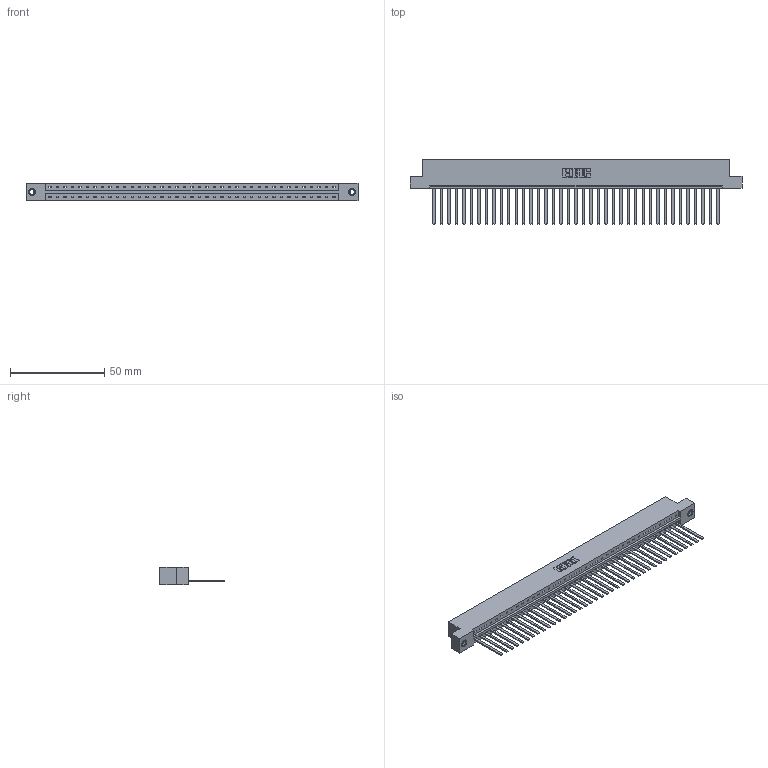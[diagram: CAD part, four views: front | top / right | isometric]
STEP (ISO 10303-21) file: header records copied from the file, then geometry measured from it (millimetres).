
FILE_DESCRIPTION (( 'STEP AP203' ), '1' );
FILE_NAME ('333-039-544-108.STEP', '2018-08-03T13:06:28', ( '' ), ( '' ), 'SwSTEP 2.0', 'SolidWorks 2016', '' );
FILE_SCHEMA (( 'CONFIG_CONTROL_DESIGN' ));
Length unit declared in the file: inch
Products named in the file (4): 333 Part_Flush - .156 Dia - TI; 345-292-001_345-293-144; 345-250-001_345-250-003-102; 333-039-544-108
Assembly tree (42 placements, depth 2):
  333-039-544-108
    333 Part_Flush - .156 Dia - TI
    345-292-001_345-293-144  x39
    345-250-001_345-250-003-102  x2
Bounding box: 176.07 x 34.3 x 9.4 mm (x, y, z)
Volume: 18137.2 mm3; surface area: 21099.1 mm2
Topology: 42 solids, 42 shells, 2202 faces, 6609 edges, 4346 vertices
Faces by surface type: plane 1584, cylinder 602, cone 12, torus 4
Entity records: 25232 total; most frequent: CARTESIAN_POINT 4334, ORIENTED_EDGE 4302, DIRECTION 3691, EDGE_CURVE 2151, LINE 2007, VECTOR 2007, VERTEX_POINT 1428, AXIS2_PLACEMENT_3D 842
